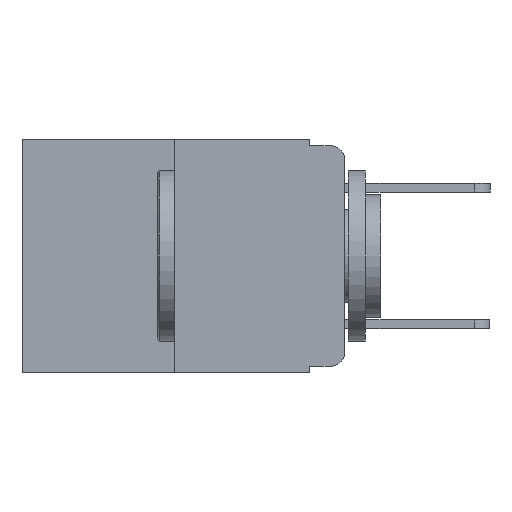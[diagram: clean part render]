
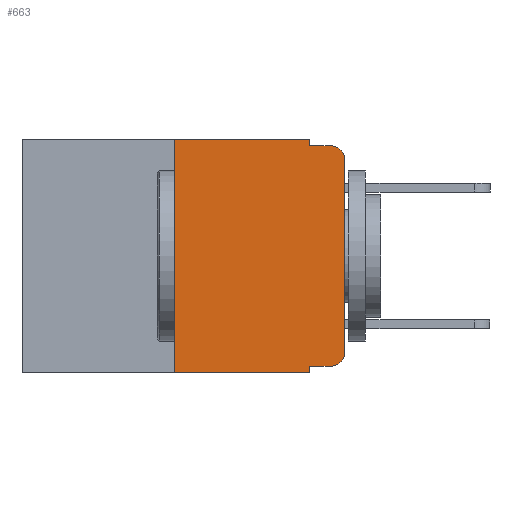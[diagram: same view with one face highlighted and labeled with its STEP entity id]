
A CAD part, left-side view. The second image highlights one B-rep face of the part: STEP entity #663.
In plain terms, the highlighted planar face has unit normal (-1, 0, 0).
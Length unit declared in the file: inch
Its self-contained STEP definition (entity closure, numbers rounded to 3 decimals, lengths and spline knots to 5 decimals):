
#80 = VERTEX_POINT ( 'NONE', #20446 ) ;
#290 = CARTESIAN_POINT ( 'NONE',  ( 0., 0.051, -0.333 ) ) ;
#511 = EDGE_CURVE ( 'NONE', #10086, #10967, #10929, .T. ) ;
#550 = VERTEX_POINT ( 'NONE', #12497 ) ;
#663 = ADVANCED_FACE ( 'NONE', ( #13394 ), #8855, .F. ) ;
#1466 = VECTOR ( 'NONE', #21450, 39.37008 ) ;
#2154 = EDGE_CURVE ( 'NONE', #2528, #10038, #15530, .T. ) ;
#2194 = CARTESIAN_POINT ( 'NONE',  ( 0., 0.051, -0.01 ) ) ;
#2401 = EDGE_CURVE ( 'NONE', #550, #7453, #5858, .T. ) ;
#2456 = VECTOR ( 'NONE', #20118, 39.37008 ) ;
#2528 = VERTEX_POINT ( 'NONE', #7772 ) ;
#2581 = CARTESIAN_POINT ( 'NONE',  ( 0., 0.25, 0. ) ) ;
#2985 = CARTESIAN_POINT ( 'NONE',  ( 0., 0.051, 0. ) ) ;
#3060 = CARTESIAN_POINT ( 'NONE',  ( 0., 0.02, -0.03 ) ) ;
#3161 = ORIENTED_EDGE ( 'NONE', *, *, #2154, .T. ) ;
#4241 = DIRECTION ( 'NONE',  ( 0., -1., 0. ) ) ;
#4814 = DIRECTION ( 'NONE',  ( 0., 0., -1. ) ) ;
#5006 = EDGE_CURVE ( 'NONE', #10086, #80, #8814, .T. ) ;
#5858 = LINE ( 'NONE', #2194, #10590 ) ;
#5861 = ORIENTED_EDGE ( 'NONE', *, *, #19259, .F. ) ;
#5890 = ORIENTED_EDGE ( 'NONE', *, *, #7330, .F. ) ;
#6163 = VECTOR ( 'NONE', #15321, 39.37008 ) ;
#6279 = CIRCLE ( 'NONE', #20291, 0.02 ) ;
#6318 = CARTESIAN_POINT ( 'NONE',  ( 0., 0., 0. ) ) ;
#6362 = CARTESIAN_POINT ( 'NONE',  ( 0., 0.02, -0.01 ) ) ;
#6872 = EDGE_CURVE ( 'NONE', #10038, #13262, #11770, .T. ) ;
#7025 = LINE ( 'NONE', #16540, #15856 ) ;
#7330 = EDGE_CURVE ( 'NONE', #2528, #10967, #7025, .T. ) ;
#7453 = VERTEX_POINT ( 'NONE', #6362 ) ;
#7772 = CARTESIAN_POINT ( 'NONE',  ( 0., 0.051, -0.333 ) ) ;
#8034 = VERTEX_POINT ( 'NONE', #21904 ) ;
#8199 = CARTESIAN_POINT ( 'NONE',  ( 0., 0.02, -0.333 ) ) ;
#8260 = VECTOR ( 'NONE', #18401, 39.37008 ) ;
#8420 = CARTESIAN_POINT ( 'NONE',  ( 0., 0.25, -0.343 ) ) ;
#8763 = DIRECTION ( 'NONE',  ( 1., 0., 0. ) ) ;
#8765 = EDGE_CURVE ( 'NONE', #17537, #550, #15542, .T. ) ;
#8811 = DIRECTION ( 'NONE',  ( 0., 0., -1. ) ) ;
#8814 = LINE ( 'NONE', #2581, #8260 ) ;
#8855 = PLANE ( 'NONE',  #15446 ) ;
#8879 = CARTESIAN_POINT ( 'NONE',  ( 0., 0.473, 0. ) ) ;
#10038 = VERTEX_POINT ( 'NONE', #8199 ) ;
#10086 = VERTEX_POINT ( 'NONE', #8420 ) ;
#10146 = CARTESIAN_POINT ( 'NONE',  ( 0., 0.02, -0.313 ) ) ;
#10373 = VECTOR ( 'NONE', #13268, 39.37008 ) ;
#10590 = VECTOR ( 'NONE', #4241, 39.37008 ) ;
#10834 = ORIENTED_EDGE ( 'NONE', *, *, #22399, .T. ) ;
#10929 = LINE ( 'NONE', #13726, #10373 ) ;
#10967 = VERTEX_POINT ( 'NONE', #21475 ) ;
#11485 = CARTESIAN_POINT ( 'NONE',  ( 0., 0.473, 0. ) ) ;
#11770 = CIRCLE ( 'NONE', #12499, 0.02 ) ;
#11843 = EDGE_CURVE ( 'NONE', #8034, #7453, #6279, .T. ) ;
#11899 = DIRECTION ( 'NONE',  ( 0., 0., -1. ) ) ;
#12497 = CARTESIAN_POINT ( 'NONE',  ( 0., 0.051, -0.01 ) ) ;
#12499 = AXIS2_PLACEMENT_3D ( 'NONE', #10146, #22264, #11899 ) ;
#12525 = ORIENTED_EDGE ( 'NONE', *, *, #8765, .F. ) ;
#13231 = ORIENTED_EDGE ( 'NONE', *, *, #6872, .T. ) ;
#13262 = VERTEX_POINT ( 'NONE', #14427 ) ;
#13268 = DIRECTION ( 'NONE',  ( 0., -1., 0. ) ) ;
#13394 = FACE_OUTER_BOUND ( 'NONE', #22329, .T. ) ;
#13395 = CARTESIAN_POINT ( 'NONE',  ( 0., 0.051, 0. ) ) ;
#13726 = CARTESIAN_POINT ( 'NONE',  ( 0., 0.473, -0.343 ) ) ;
#13896 = LINE ( 'NONE', #6318, #21988 ) ;
#14427 = CARTESIAN_POINT ( 'NONE',  ( 0., 0., -0.313 ) ) ;
#15321 = DIRECTION ( 'NONE',  ( 0., 0., -1. ) ) ;
#15386 = DIRECTION ( 'NONE',  ( -1., 0., 0. ) ) ;
#15446 = AXIS2_PLACEMENT_3D ( 'NONE', #8879, #8763, #8811 ) ;
#15530 = LINE ( 'NONE', #290, #1466 ) ;
#15542 = LINE ( 'NONE', #2985, #6163 ) ;
#15856 = VECTOR ( 'NONE', #18293, 39.37008 ) ;
#16540 = CARTESIAN_POINT ( 'NONE',  ( 0., 0.051, 0. ) ) ;
#16634 = ORIENTED_EDGE ( 'NONE', *, *, #511, .T. ) ;
#17537 = VERTEX_POINT ( 'NONE', #13395 ) ;
#18293 = DIRECTION ( 'NONE',  ( 0., 0., -1. ) ) ;
#18401 = DIRECTION ( 'NONE',  ( 0., 0., 1. ) ) ;
#18505 = ORIENTED_EDGE ( 'NONE', *, *, #2401, .F. ) ;
#19259 = EDGE_CURVE ( 'NONE', #80, #17537, #21052, .T. ) ;
#20118 = DIRECTION ( 'NONE',  ( 0., -1., 0. ) ) ;
#20291 = AXIS2_PLACEMENT_3D ( 'NONE', #3060, #15386, #4814 ) ;
#20313 = DIRECTION ( 'NONE',  ( 0., 0., 1. ) ) ;
#20344 = ORIENTED_EDGE ( 'NONE', *, *, #11843, .T. ) ;
#20446 = CARTESIAN_POINT ( 'NONE',  ( 0., 0.25, 0. ) ) ;
#21052 = LINE ( 'NONE', #11485, #2456 ) ;
#21450 = DIRECTION ( 'NONE',  ( 0., -1., 0. ) ) ;
#21475 = CARTESIAN_POINT ( 'NONE',  ( 0., 0.051, -0.343 ) ) ;
#21904 = CARTESIAN_POINT ( 'NONE',  ( 0., 0., -0.03 ) ) ;
#21984 = ORIENTED_EDGE ( 'NONE', *, *, #5006, .F. ) ;
#21988 = VECTOR ( 'NONE', #20313, 39.37008 ) ;
#22264 = DIRECTION ( 'NONE',  ( -1., 0., 0. ) ) ;
#22329 = EDGE_LOOP ( 'NONE', ( #10834, #20344, #18505, #12525, #5861, #21984, #16634, #5890, #3161, #13231 ) ) ;
#22399 = EDGE_CURVE ( 'NONE', #13262, #8034, #13896, .T. ) ;
